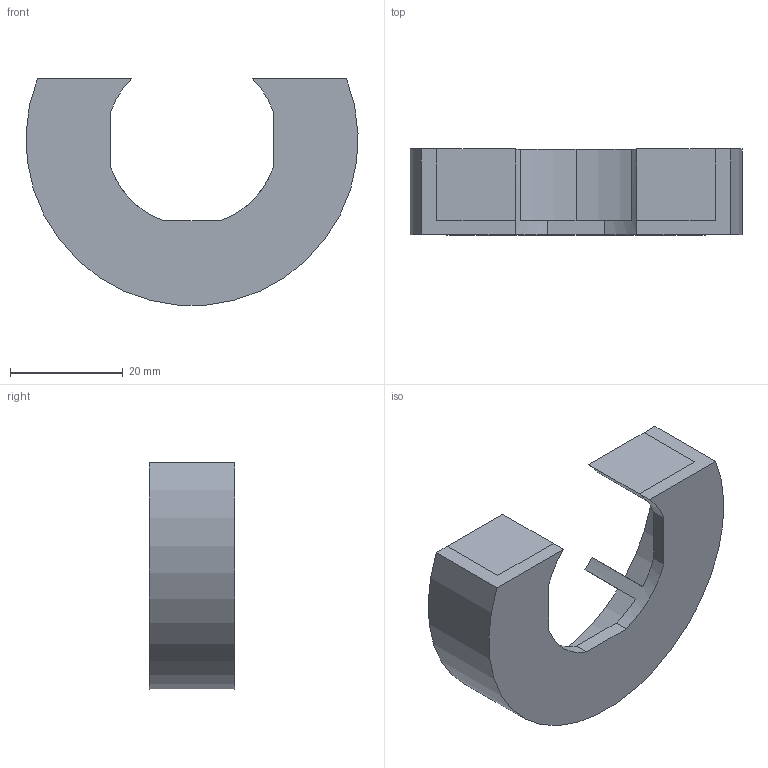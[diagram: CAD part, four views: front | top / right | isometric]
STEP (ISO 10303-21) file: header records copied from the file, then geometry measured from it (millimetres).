
FILE_DESCRIPTION (( 'STEP AP214' ), '1' );
FILE_NAME ('chamber.STEP', '2013-07-04T02:22:50', ( '' ), ( '' ), 'SwSTEP 2.0', 'SolidWorks 2012', '' );
FILE_SCHEMA (( 'AUTOMOTIVE_DESIGN' ));
Length unit declared in the file: inch
Products named in the file (1): chamber
Bounding box: 58.95 x 15.24 x 40.18 mm (x, y, z)
Volume: 8602.8 mm3; surface area: 7688.6 mm2
Topology: 3 solids, 3 shells, 37 faces, 93 edges, 62 vertices
Faces by surface type: plane 24, cylinder 13
Entity records: 1179 total; most frequent: DIRECTION 199, CARTESIAN_POINT 193, ORIENTED_EDGE 186, EDGE_CURVE 93, AXIS2_PLACEMENT_3D 68, VECTOR 63, LINE 63, VERTEX_POINT 62
